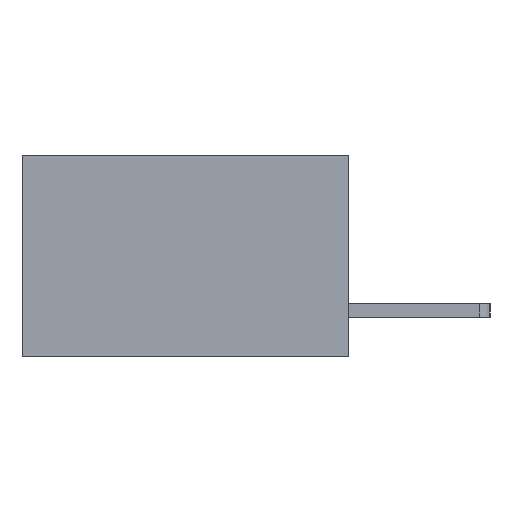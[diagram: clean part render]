
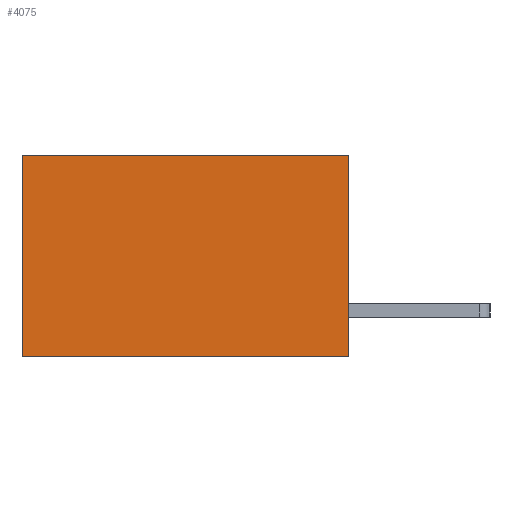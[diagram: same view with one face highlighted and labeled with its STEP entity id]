
A CAD part, left-side view. The second image highlights one B-rep face of the part: STEP entity #4075.
In plain terms, the highlighted planar face has unit normal (-1, 0, 0).
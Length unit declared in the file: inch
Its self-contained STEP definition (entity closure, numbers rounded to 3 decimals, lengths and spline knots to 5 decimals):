
#228 = ORIENTED_EDGE ( 'NONE', *, *, #1575, .T. ) ;
#319 = VECTOR ( 'NONE', #2731, 39.37008 ) ;
#492 = DIRECTION ( 'NONE',  ( 0., 1., 0. ) ) ;
#722 = ORIENTED_EDGE ( 'NONE', *, *, #1301, .F. ) ;
#976 = DIRECTION ( 'NONE',  ( 0., 0., -1. ) ) ;
#978 = ORIENTED_EDGE ( 'NONE', *, *, #1951, .F. ) ;
#1301 = EDGE_CURVE ( 'NONE', #4871, #3667, #7088, .T. ) ;
#1575 = EDGE_CURVE ( 'NONE', #4871, #6769, #4322, .T. ) ;
#1897 = VECTOR ( 'NONE', #976, 39.37008 ) ;
#1951 = EDGE_CURVE ( 'NONE', #3667, #9726, #6845, .T. ) ;
#2013 = VECTOR ( 'NONE', #3579, 39.37008 ) ;
#2016 = EDGE_CURVE ( 'NONE', #6769, #9726, #8549, .T. ) ;
#2731 = DIRECTION ( 'NONE',  ( 0., 0., -1. ) ) ;
#2918 = CARTESIAN_POINT ( 'NONE',  ( 0.2615, 0.6, -0.37 ) ) ;
#2926 = CARTESIAN_POINT ( 'NONE',  ( 0.2615, 0., 0. ) ) ;
#2954 = DIRECTION ( 'NONE',  ( 0., 0., -1. ) ) ;
#2967 = DIRECTION ( 'NONE',  ( 1., 0., 0. ) ) ;
#2979 = PLANE ( 'NONE',  #6900 ) ;
#3158 = CARTESIAN_POINT ( 'NONE',  ( 0.2615, 0., -0.37 ) ) ;
#3579 = DIRECTION ( 'NONE',  ( 0., 1., 0. ) ) ;
#3667 = VERTEX_POINT ( 'NONE', #8196 ) ;
#3945 = CARTESIAN_POINT ( 'NONE',  ( 0.2615, 0.6, -0.37 ) ) ;
#4075 = ADVANCED_FACE ( 'NONE', ( #4412 ), #2979, .F. ) ;
#4322 = LINE ( 'NONE', #2926, #2013 ) ;
#4412 = FACE_OUTER_BOUND ( 'NONE', #9257, .T. ) ;
#4740 = VECTOR ( 'NONE', #492, 39.37008 ) ;
#4871 = VERTEX_POINT ( 'NONE', #6111 ) ;
#5585 = CARTESIAN_POINT ( 'NONE',  ( 0.2615, 0., -0.37 ) ) ;
#6100 = CARTESIAN_POINT ( 'NONE',  ( 0.2615, 0., -0.37 ) ) ;
#6111 = CARTESIAN_POINT ( 'NONE',  ( 0.2615, 0., 0. ) ) ;
#6769 = VERTEX_POINT ( 'NONE', #8953 ) ;
#6845 = LINE ( 'NONE', #6100, #4740 ) ;
#6900 = AXIS2_PLACEMENT_3D ( 'NONE', #3158, #2967, #2954 ) ;
#7088 = LINE ( 'NONE', #5585, #319 ) ;
#7405 = ORIENTED_EDGE ( 'NONE', *, *, #2016, .T. ) ;
#8196 = CARTESIAN_POINT ( 'NONE',  ( 0.2615, 0., -0.37 ) ) ;
#8549 = LINE ( 'NONE', #2918, #1897 ) ;
#8953 = CARTESIAN_POINT ( 'NONE',  ( 0.2615, 0.6, 0. ) ) ;
#9257 = EDGE_LOOP ( 'NONE', ( #7405, #978, #722, #228 ) ) ;
#9726 = VERTEX_POINT ( 'NONE', #3945 ) ;
